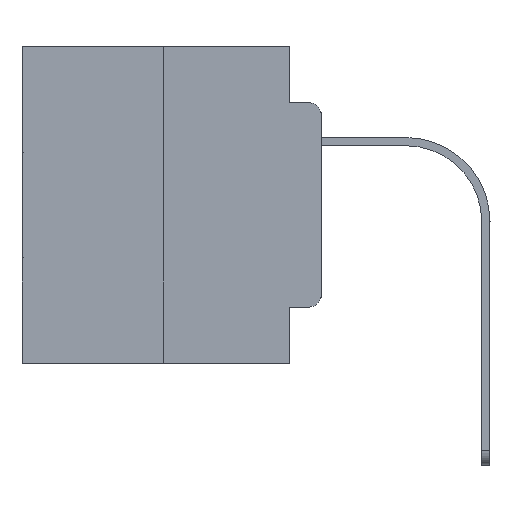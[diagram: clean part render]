
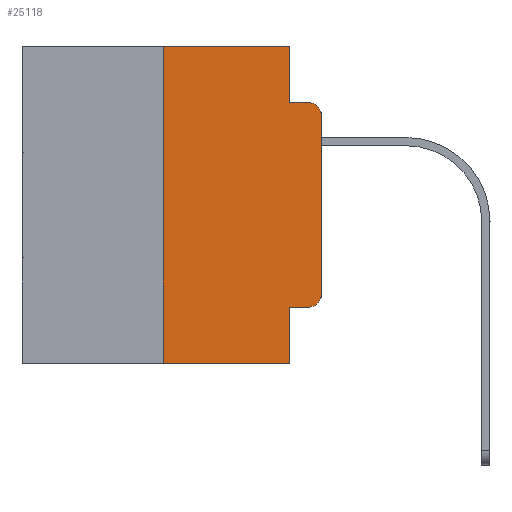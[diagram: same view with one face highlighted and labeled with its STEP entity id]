
A CAD part, left-side view. The second image highlights one B-rep face of the part: STEP entity #25118.
In plain terms, the highlighted planar face has unit normal (-1, 0, 0).
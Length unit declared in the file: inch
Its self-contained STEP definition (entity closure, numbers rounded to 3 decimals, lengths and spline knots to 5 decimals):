
#21 = VERTEX_POINT ( 'NONE', #21011 ) ;
#306 = VERTEX_POINT ( 'NONE', #3122 ) ;
#312 = DIRECTION ( 'NONE',  ( 1., 0., 0. ) ) ;
#324 = EDGE_CURVE ( 'NONE', #17254, #10011, #11841, .T. ) ;
#820 = PLANE ( 'NONE',  #17462 ) ;
#874 = VECTOR ( 'NONE', #11639, 39.37008 ) ;
#1036 = CIRCLE ( 'NONE', #23583, 0.02 ) ;
#1331 = CARTESIAN_POINT ( 'NONE',  ( 0., 0.473, -0.5 ) ) ;
#1387 = CARTESIAN_POINT ( 'NONE',  ( 0., 0.02, -0.4115 ) ) ;
#1608 = AXIS2_PLACEMENT_3D ( 'NONE', #2862, #6863, #6591 ) ;
#1689 = CARTESIAN_POINT ( 'NONE',  ( 0., 0.051, 0. ) ) ;
#2296 = CARTESIAN_POINT ( 'NONE',  ( 0., 0.051, -0.0885 ) ) ;
#2862 = CARTESIAN_POINT ( 'NONE',  ( 0., 0.02, -0.1085 ) ) ;
#3122 = CARTESIAN_POINT ( 'NONE',  ( 0., 0.02, -0.0885 ) ) ;
#3367 = VERTEX_POINT ( 'NONE', #20940 ) ;
#4708 = CARTESIAN_POINT ( 'NONE',  ( 0., 0.051, -0.5 ) ) ;
#4715 = CARTESIAN_POINT ( 'NONE',  ( 0., 0.051, -0.0885 ) ) ;
#4785 = VECTOR ( 'NONE', #11846, 39.37008 ) ;
#4952 = CARTESIAN_POINT ( 'NONE',  ( 0., 0.473, 0. ) ) ;
#5052 = ORIENTED_EDGE ( 'NONE', *, *, #14814, .T. ) ;
#5505 = LINE ( 'NONE', #7848, #9450 ) ;
#5664 = DIRECTION ( 'NONE',  ( 0., 0., 1. ) ) ;
#5695 = VECTOR ( 'NONE', #8697, 39.37008 ) ;
#6346 = EDGE_CURVE ( 'NONE', #17254, #21801, #9841, .T. ) ;
#6348 = CARTESIAN_POINT ( 'NONE',  ( 0., 0.051, 0. ) ) ;
#6591 = DIRECTION ( 'NONE',  ( 0., 0., -1. ) ) ;
#6621 = DIRECTION ( 'NONE',  ( 0., 0., -1. ) ) ;
#6863 = DIRECTION ( 'NONE',  ( -1., 0., 0. ) ) ;
#7488 = DIRECTION ( 'NONE',  ( 0., 0., -1. ) ) ;
#7633 = CARTESIAN_POINT ( 'NONE',  ( 0., 0.25, 0. ) ) ;
#7807 = ORIENTED_EDGE ( 'NONE', *, *, #6346, .F. ) ;
#7848 = CARTESIAN_POINT ( 'NONE',  ( 0., 0., 0. ) ) ;
#7932 = ORIENTED_EDGE ( 'NONE', *, *, #21241, .T. ) ;
#8366 = CARTESIAN_POINT ( 'NONE',  ( 0., 0.25, 0. ) ) ;
#8697 = DIRECTION ( 'NONE',  ( 0., 0., -1. ) ) ;
#9357 = DIRECTION ( 'NONE',  ( 0., -1., 0. ) ) ;
#9450 = VECTOR ( 'NONE', #24909, 39.37008 ) ;
#9841 = LINE ( 'NONE', #7633, #23860 ) ;
#10011 = VERTEX_POINT ( 'NONE', #4708 ) ;
#10074 = VERTEX_POINT ( 'NONE', #1387 ) ;
#10459 = CIRCLE ( 'NONE', #1608, 0.02 ) ;
#11047 = VECTOR ( 'NONE', #15163, 39.37008 ) ;
#11562 = EDGE_LOOP ( 'NONE', ( #7932, #14954, #18188, #20765, #21088, #7807, #17976, #20708, #12386, #5052 ) ) ;
#11639 = DIRECTION ( 'NONE',  ( 0., -1., 0. ) ) ;
#11841 = LINE ( 'NONE', #1331, #22720 ) ;
#11846 = DIRECTION ( 'NONE',  ( 0., -1., 0. ) ) ;
#12386 = ORIENTED_EDGE ( 'NONE', *, *, #21775, .T. ) ;
#12449 = EDGE_CURVE ( 'NONE', #15355, #27229, #19755, .T. ) ;
#12513 = VERTEX_POINT ( 'NONE', #16433 ) ;
#13320 = LINE ( 'NONE', #4715, #874 ) ;
#14814 = EDGE_CURVE ( 'NONE', #10074, #21, #1036, .T. ) ;
#14954 = ORIENTED_EDGE ( 'NONE', *, *, #26793, .T. ) ;
#15163 = DIRECTION ( 'NONE',  ( 0., -1., 0. ) ) ;
#15355 = VERTEX_POINT ( 'NONE', #1689 ) ;
#15612 = EDGE_CURVE ( 'NONE', #27229, #306, #13320, .T. ) ;
#15932 = EDGE_CURVE ( 'NONE', #3367, #10011, #25192, .T. ) ;
#16433 = CARTESIAN_POINT ( 'NONE',  ( 0., 0., -0.1085 ) ) ;
#17254 = VERTEX_POINT ( 'NONE', #24073 ) ;
#17380 = LINE ( 'NONE', #25802, #11047 ) ;
#17462 = AXIS2_PLACEMENT_3D ( 'NONE', #4952, #312, #6621 ) ;
#17818 = CARTESIAN_POINT ( 'NONE',  ( 0., 0.051, 0. ) ) ;
#17976 = ORIENTED_EDGE ( 'NONE', *, *, #324, .T. ) ;
#18012 = DIRECTION ( 'NONE',  ( -1., 0., 0. ) ) ;
#18188 = ORIENTED_EDGE ( 'NONE', *, *, #15612, .F. ) ;
#19755 = LINE ( 'NONE', #17818, #25818 ) ;
#20708 = ORIENTED_EDGE ( 'NONE', *, *, #15932, .F. ) ;
#20765 = ORIENTED_EDGE ( 'NONE', *, *, #12449, .F. ) ;
#20940 = CARTESIAN_POINT ( 'NONE',  ( 0., 0.051, -0.4115 ) ) ;
#21011 = CARTESIAN_POINT ( 'NONE',  ( 0., 0., -0.3915 ) ) ;
#21088 = ORIENTED_EDGE ( 'NONE', *, *, #21907, .F. ) ;
#21241 = EDGE_CURVE ( 'NONE', #21, #12513, #5505, .T. ) ;
#21775 = EDGE_CURVE ( 'NONE', #3367, #10074, #22388, .T. ) ;
#21801 = VERTEX_POINT ( 'NONE', #8366 ) ;
#21907 = EDGE_CURVE ( 'NONE', #21801, #15355, #17380, .T. ) ;
#22388 = LINE ( 'NONE', #24453, #4785 ) ;
#22720 = VECTOR ( 'NONE', #9357, 39.37008 ) ;
#23543 = FACE_OUTER_BOUND ( 'NONE', #11562, .T. ) ;
#23583 = AXIS2_PLACEMENT_3D ( 'NONE', #26593, #18012, #7488 ) ;
#23860 = VECTOR ( 'NONE', #5664, 39.37008 ) ;
#24073 = CARTESIAN_POINT ( 'NONE',  ( 0., 0.25, -0.5 ) ) ;
#24453 = CARTESIAN_POINT ( 'NONE',  ( 0., 0.051, -0.4115 ) ) ;
#24879 = DIRECTION ( 'NONE',  ( 0., 0., -1. ) ) ;
#24909 = DIRECTION ( 'NONE',  ( 0., 0., 1. ) ) ;
#25118 = ADVANCED_FACE ( 'NONE', ( #23543 ), #820, .F. ) ;
#25192 = LINE ( 'NONE', #6348, #5695 ) ;
#25802 = CARTESIAN_POINT ( 'NONE',  ( 0., 0.473, 0. ) ) ;
#25818 = VECTOR ( 'NONE', #24879, 39.37008 ) ;
#26593 = CARTESIAN_POINT ( 'NONE',  ( 0., 0.02, -0.3915 ) ) ;
#26793 = EDGE_CURVE ( 'NONE', #12513, #306, #10459, .T. ) ;
#27229 = VERTEX_POINT ( 'NONE', #2296 ) ;
